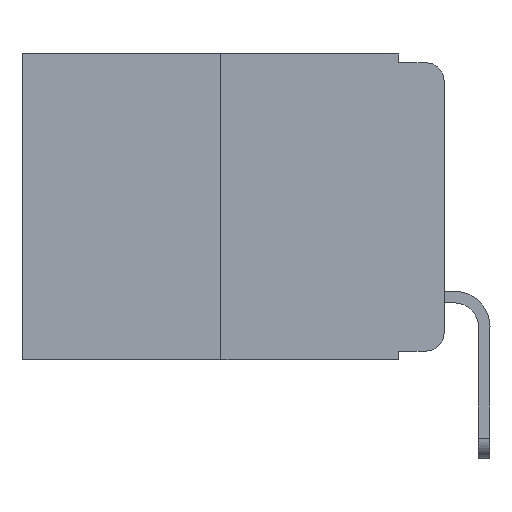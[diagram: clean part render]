
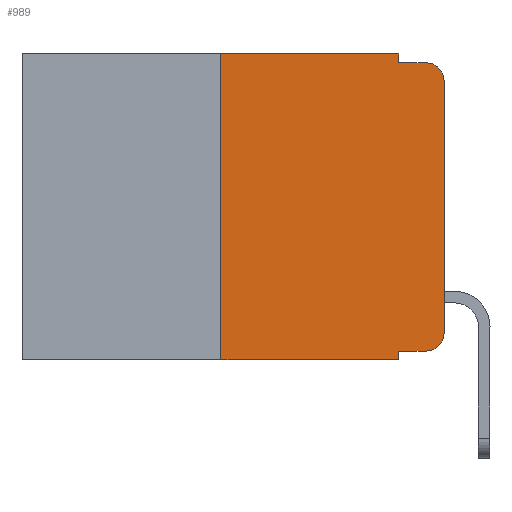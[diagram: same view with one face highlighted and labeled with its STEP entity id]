
A CAD part, left-side view. The second image highlights one B-rep face of the part: STEP entity #989.
In plain terms, the highlighted planar face has unit normal (-1, 0, 0).
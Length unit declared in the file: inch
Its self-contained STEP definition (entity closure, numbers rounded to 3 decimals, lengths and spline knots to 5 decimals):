
#212 = CARTESIAN_POINT ( 'NONE',  ( 0., 0.051, 0. ) ) ;
#263 = DIRECTION ( 'NONE',  ( 0., 0., -1. ) ) ;
#322 = LINE ( 'NONE', #16406, #18583 ) ;
#467 = CARTESIAN_POINT ( 'NONE',  ( 0., 0.02, -0.01 ) ) ;
#989 = ADVANCED_FACE ( 'NONE', ( #6014 ), #7953, .F. ) ;
#1316 = ORIENTED_EDGE ( 'NONE', *, *, #7704, .T. ) ;
#1590 = ORIENTED_EDGE ( 'NONE', *, *, #4433, .F. ) ;
#1643 = ORIENTED_EDGE ( 'NONE', *, *, #10939, .T. ) ;
#1934 = DIRECTION ( 'NONE',  ( 0., 0., 1. ) ) ;
#2141 = CARTESIAN_POINT ( 'NONE',  ( 0., 0.051, -0.333 ) ) ;
#2301 = EDGE_CURVE ( 'NONE', #3800, #15711, #16641, .T. ) ;
#2801 = CARTESIAN_POINT ( 'NONE',  ( 0., 0., 0. ) ) ;
#3223 = LINE ( 'NONE', #3511, #6209 ) ;
#3394 = AXIS2_PLACEMENT_3D ( 'NONE', #9555, #4904, #6474 ) ;
#3511 = CARTESIAN_POINT ( 'NONE',  ( 0., 0.051, 0. ) ) ;
#3800 = VERTEX_POINT ( 'NONE', #12506 ) ;
#4205 = VERTEX_POINT ( 'NONE', #18132 ) ;
#4433 = EDGE_CURVE ( 'NONE', #18458, #6058, #3223, .T. ) ;
#4904 = DIRECTION ( 'NONE',  ( 1., 0., 0. ) ) ;
#5669 = DIRECTION ( 'NONE',  ( 0., -1., 0. ) ) ;
#6014 = FACE_OUTER_BOUND ( 'NONE', #8210, .T. ) ;
#6058 = VERTEX_POINT ( 'NONE', #16624 ) ;
#6092 = ORIENTED_EDGE ( 'NONE', *, *, #11300, .T. ) ;
#6209 = VECTOR ( 'NONE', #16283, 39.37008 ) ;
#6346 = DIRECTION ( 'NONE',  ( -1., 0., 0. ) ) ;
#6430 = CARTESIAN_POINT ( 'NONE',  ( 0., 0.25, 0. ) ) ;
#6474 = DIRECTION ( 'NONE',  ( 0., 0., -1. ) ) ;
#6947 = DIRECTION ( 'NONE',  ( 0., 0., -1. ) ) ;
#7261 = VECTOR ( 'NONE', #15245, 39.37008 ) ;
#7666 = CARTESIAN_POINT ( 'NONE',  ( 0., 0.051, -0.01 ) ) ;
#7698 = VERTEX_POINT ( 'NONE', #467 ) ;
#7704 = EDGE_CURVE ( 'NONE', #15711, #7698, #16239, .T. ) ;
#7884 = VECTOR ( 'NONE', #1934, 39.37008 ) ;
#7953 = PLANE ( 'NONE',  #3394 ) ;
#8092 = CARTESIAN_POINT ( 'NONE',  ( 0., 0.473, 0. ) ) ;
#8210 = EDGE_LOOP ( 'NONE', ( #11094, #1316, #15709, #9069, #10689, #17245, #6092, #1590, #17848, #1643 ) ) ;
#8339 = LINE ( 'NONE', #12019, #11556 ) ;
#8606 = CIRCLE ( 'NONE', #16257, 0.02 ) ;
#9069 = ORIENTED_EDGE ( 'NONE', *, *, #9966, .F. ) ;
#9091 = CARTESIAN_POINT ( 'NONE',  ( 0., 0.051, -0.01 ) ) ;
#9278 = CARTESIAN_POINT ( 'NONE',  ( 0., 0.02, -0.313 ) ) ;
#9555 = CARTESIAN_POINT ( 'NONE',  ( 0., 0.473, 0. ) ) ;
#9765 = LINE ( 'NONE', #212, #11746 ) ;
#9852 = VERTEX_POINT ( 'NONE', #12807 ) ;
#9966 = EDGE_CURVE ( 'NONE', #9852, #15126, #9765, .T. ) ;
#10372 = LINE ( 'NONE', #7666, #13342 ) ;
#10689 = ORIENTED_EDGE ( 'NONE', *, *, #15382, .F. ) ;
#10778 = DIRECTION ( 'NONE',  ( 0., -1., 0. ) ) ;
#10939 = EDGE_CURVE ( 'NONE', #4205, #3800, #8606, .T. ) ;
#11094 = ORIENTED_EDGE ( 'NONE', *, *, #2301, .T. ) ;
#11300 = EDGE_CURVE ( 'NONE', #14923, #6058, #8339, .T. ) ;
#11497 = VERTEX_POINT ( 'NONE', #14608 ) ;
#11556 = VECTOR ( 'NONE', #18353, 39.37008 ) ;
#11746 = VECTOR ( 'NONE', #263, 39.37008 ) ;
#11891 = VECTOR ( 'NONE', #19078, 39.37008 ) ;
#12019 = CARTESIAN_POINT ( 'NONE',  ( 0., 0.473, -0.343 ) ) ;
#12506 = CARTESIAN_POINT ( 'NONE',  ( 0., 0., -0.313 ) ) ;
#12771 = AXIS2_PLACEMENT_3D ( 'NONE', #19073, #14566, #6947 ) ;
#12807 = CARTESIAN_POINT ( 'NONE',  ( 0., 0.051, 0. ) ) ;
#13342 = VECTOR ( 'NONE', #10778, 39.37008 ) ;
#14281 = EDGE_CURVE ( 'NONE', #18458, #4205, #322, .T. ) ;
#14566 = DIRECTION ( 'NONE',  ( -1., 0., 0. ) ) ;
#14608 = CARTESIAN_POINT ( 'NONE',  ( 0., 0.25, 0. ) ) ;
#14923 = VERTEX_POINT ( 'NONE', #17778 ) ;
#15126 = VERTEX_POINT ( 'NONE', #9091 ) ;
#15245 = DIRECTION ( 'NONE',  ( 0., 0., 1. ) ) ;
#15382 = EDGE_CURVE ( 'NONE', #11497, #9852, #16099, .T. ) ;
#15709 = ORIENTED_EDGE ( 'NONE', *, *, #16338, .F. ) ;
#15711 = VERTEX_POINT ( 'NONE', #18368 ) ;
#16099 = LINE ( 'NONE', #8092, #11891 ) ;
#16239 = CIRCLE ( 'NONE', #12771, 0.02 ) ;
#16257 = AXIS2_PLACEMENT_3D ( 'NONE', #9278, #6346, #17338 ) ;
#16283 = DIRECTION ( 'NONE',  ( 0., 0., -1. ) ) ;
#16338 = EDGE_CURVE ( 'NONE', #15126, #7698, #10372, .T. ) ;
#16406 = CARTESIAN_POINT ( 'NONE',  ( 0., 0.051, -0.333 ) ) ;
#16624 = CARTESIAN_POINT ( 'NONE',  ( 0., 0.051, -0.343 ) ) ;
#16641 = LINE ( 'NONE', #2801, #7261 ) ;
#17074 = EDGE_CURVE ( 'NONE', #14923, #11497, #19485, .T. ) ;
#17245 = ORIENTED_EDGE ( 'NONE', *, *, #17074, .F. ) ;
#17338 = DIRECTION ( 'NONE',  ( 0., 0., -1. ) ) ;
#17778 = CARTESIAN_POINT ( 'NONE',  ( 0., 0.25, -0.343 ) ) ;
#17848 = ORIENTED_EDGE ( 'NONE', *, *, #14281, .T. ) ;
#18132 = CARTESIAN_POINT ( 'NONE',  ( 0., 0.02, -0.333 ) ) ;
#18353 = DIRECTION ( 'NONE',  ( 0., -1., 0. ) ) ;
#18368 = CARTESIAN_POINT ( 'NONE',  ( 0., 0., -0.03 ) ) ;
#18458 = VERTEX_POINT ( 'NONE', #2141 ) ;
#18583 = VECTOR ( 'NONE', #5669, 39.37008 ) ;
#19073 = CARTESIAN_POINT ( 'NONE',  ( 0., 0.02, -0.03 ) ) ;
#19078 = DIRECTION ( 'NONE',  ( 0., -1., 0. ) ) ;
#19485 = LINE ( 'NONE', #6430, #7884 ) ;
